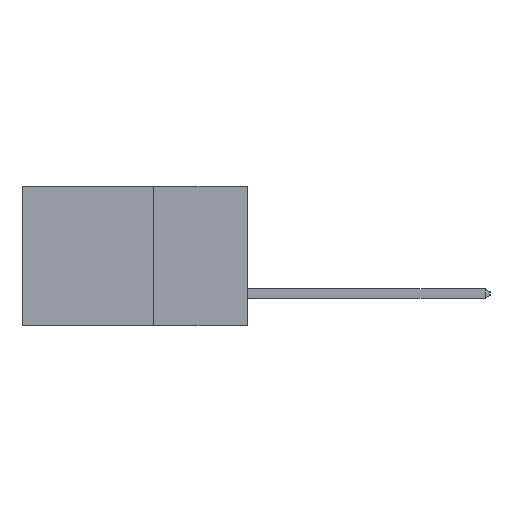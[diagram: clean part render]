
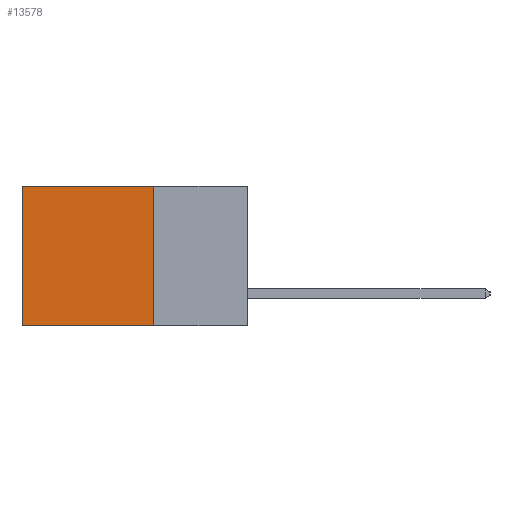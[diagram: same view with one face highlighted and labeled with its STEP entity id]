
A CAD part, left-side view. The second image highlights one B-rep face of the part: STEP entity #13578.
In plain terms, the highlighted planar face has unit normal (-1, 0, 0).
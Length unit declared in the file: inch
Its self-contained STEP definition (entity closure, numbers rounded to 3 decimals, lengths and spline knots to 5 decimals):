
#107 = DIRECTION ( 'NONE',  ( 0., 0., -1. ) ) ;
#589 = VECTOR ( 'NONE', #107, 39.37008 ) ;
#885 = VERTEX_POINT ( 'NONE', #11853 ) ;
#1162 = LINE ( 'NONE', #14383, #10534 ) ;
#1371 = DIRECTION ( 'NONE',  ( 0., 0., -1. ) ) ;
#3107 = CARTESIAN_POINT ( 'NONE',  ( 0.2615, 0.6, 0. ) ) ;
#3166 = LINE ( 'NONE', #7557, #589 ) ;
#3793 = VERTEX_POINT ( 'NONE', #7610 ) ;
#3847 = VERTEX_POINT ( 'NONE', #3107 ) ;
#4772 = VERTEX_POINT ( 'NONE', #8458 ) ;
#4912 = DIRECTION ( 'NONE',  ( 0., 0., -1. ) ) ;
#5136 = AXIS2_PLACEMENT_3D ( 'NONE', #12237, #8729, #1371 ) ;
#5442 = EDGE_CURVE ( 'NONE', #3793, #885, #8042, .T. ) ;
#6127 = CARTESIAN_POINT ( 'NONE',  ( 0.2615, 0.25, -0.37 ) ) ;
#7241 = FACE_OUTER_BOUND ( 'NONE', #12609, .T. ) ;
#7542 = PLANE ( 'NONE',  #5136 ) ;
#7557 = CARTESIAN_POINT ( 'NONE',  ( 0.2615, 0.25, -0.37 ) ) ;
#7610 = CARTESIAN_POINT ( 'NONE',  ( 0.2615, 0.25, -0.37 ) ) ;
#8042 = LINE ( 'NONE', #6127, #14290 ) ;
#8458 = CARTESIAN_POINT ( 'NONE',  ( 0.2615, 0.25, 0. ) ) ;
#8527 = ORIENTED_EDGE ( 'NONE', *, *, #5442, .F. ) ;
#8530 = DIRECTION ( 'NONE',  ( 0., 1., 0. ) ) ;
#8729 = DIRECTION ( 'NONE',  ( 1., 0., 0. ) ) ;
#9835 = ORIENTED_EDGE ( 'NONE', *, *, #10758, .T. ) ;
#10534 = VECTOR ( 'NONE', #8530, 39.37008 ) ;
#10747 = ORIENTED_EDGE ( 'NONE', *, *, #14882, .F. ) ;
#10758 = EDGE_CURVE ( 'NONE', #3847, #885, #15383, .T. ) ;
#11582 = VECTOR ( 'NONE', #4912, 39.37008 ) ;
#11853 = CARTESIAN_POINT ( 'NONE',  ( 0.2615, 0.6, -0.37 ) ) ;
#12237 = CARTESIAN_POINT ( 'NONE',  ( 0.2615, 0.25, -0.37 ) ) ;
#12609 = EDGE_LOOP ( 'NONE', ( #9835, #8527, #10747, #15287 ) ) ;
#13215 = CARTESIAN_POINT ( 'NONE',  ( 0.2615, 0.6, -0.37 ) ) ;
#13578 = ADVANCED_FACE ( 'NONE', ( #7241 ), #7542, .F. ) ;
#14290 = VECTOR ( 'NONE', #14387, 39.37008 ) ;
#14383 = CARTESIAN_POINT ( 'NONE',  ( 0.2615, 0.25, 0. ) ) ;
#14387 = DIRECTION ( 'NONE',  ( 0., 1., 0. ) ) ;
#14882 = EDGE_CURVE ( 'NONE', #4772, #3793, #3166, .T. ) ;
#15287 = ORIENTED_EDGE ( 'NONE', *, *, #15401, .T. ) ;
#15383 = LINE ( 'NONE', #13215, #11582 ) ;
#15401 = EDGE_CURVE ( 'NONE', #4772, #3847, #1162, .T. ) ;
